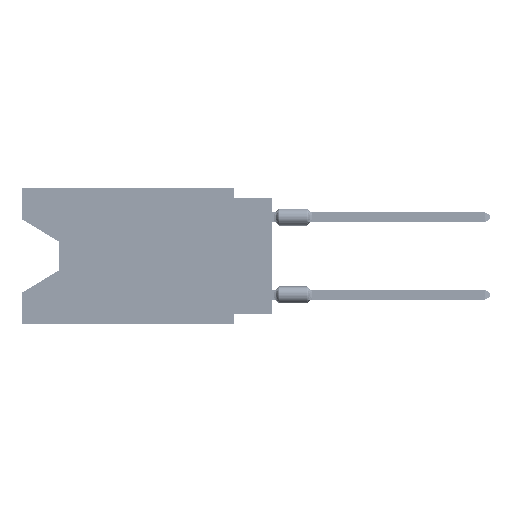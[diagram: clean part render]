
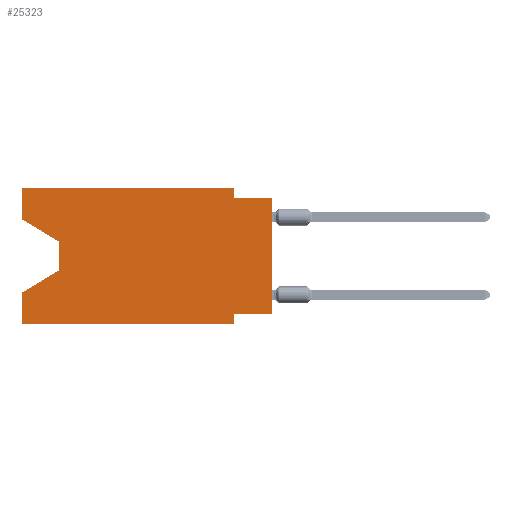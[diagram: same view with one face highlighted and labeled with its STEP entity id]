
A CAD part, left-side view. The second image highlights one B-rep face of the part: STEP entity #25323.
In plain terms, the highlighted planar face has unit normal (-1, 0, 0).
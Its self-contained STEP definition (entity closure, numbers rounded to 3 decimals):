
#1322 = DIRECTION ( 'NONE',  ( 0., -1., 0. ) ) ;
#2006 = CARTESIAN_POINT ( 'NONE',  ( 0., 2.54, -8.89 ) ) ;
#2215 = ORIENTED_EDGE ( 'NONE', *, *, #45818, .F. ) ;
#2625 = VECTOR ( 'NONE', #82214, 1000. ) ;
#3674 = CARTESIAN_POINT ( 'NONE',  ( 0., 16.383, -6.852 ) ) ;
#5440 = ORIENTED_EDGE ( 'NONE', *, *, #59265, .F. ) ;
#5467 = DIRECTION ( 'NONE',  ( 0., 0., -1. ) ) ;
#6270 = CARTESIAN_POINT ( 'NONE',  ( 0., 13.97, -3.505 ) ) ;
#6957 = VERTEX_POINT ( 'NONE', #6270 ) ;
#7101 = LINE ( 'NONE', #88736, #16648 ) ;
#7112 = LINE ( 'NONE', #82929, #27342 ) ;
#7454 = ORIENTED_EDGE ( 'NONE', *, *, #74596, .T. ) ;
#8491 = ORIENTED_EDGE ( 'NONE', *, *, #35704, .T. ) ;
#8925 = VERTEX_POINT ( 'NONE', #3674 ) ;
#10332 = CARTESIAN_POINT ( 'NONE',  ( 0., 16.383, -8.89 ) ) ;
#14227 = CARTESIAN_POINT ( 'NONE',  ( 0., 0., -8.255 ) ) ;
#15724 = VERTEX_POINT ( 'NONE', #23670 ) ;
#15824 = LINE ( 'NONE', #31757, #81781 ) ;
#16503 = LINE ( 'NONE', #47361, #63998 ) ;
#16648 = VECTOR ( 'NONE', #44758, 1000. ) ;
#17114 = ORIENTED_EDGE ( 'NONE', *, *, #38136, .F. ) ;
#20661 = ORIENTED_EDGE ( 'NONE', *, *, #65921, .T. ) ;
#21533 = EDGE_CURVE ( 'NONE', #89520, #93543, #53002, .T. ) ;
#22198 = ORIENTED_EDGE ( 'NONE', *, *, #42359, .F. ) ;
#23315 = EDGE_CURVE ( 'NONE', #33193, #8925, #7101, .T. ) ;
#23670 = CARTESIAN_POINT ( 'NONE',  ( 0., 16.383, 0. ) ) ;
#23879 = EDGE_LOOP ( 'NONE', ( #20661, #61763, #7454, #28850, #8491, #17114, #90145, #60807, #91221, #2215, #5440, #22198 ) ) ;
#24011 = DIRECTION ( 'NONE',  ( 0., 1., 0. ) ) ;
#24727 = VERTEX_POINT ( 'NONE', #70320 ) ;
#24990 = CARTESIAN_POINT ( 'NONE',  ( 0., 2.54, -8.255 ) ) ;
#25323 = ADVANCED_FACE ( 'NONE', ( #49422 ), #42177, .F. ) ;
#26216 = CARTESIAN_POINT ( 'NONE',  ( 0., 0., 0. ) ) ;
#27342 = VECTOR ( 'NONE', #24011, 1000. ) ;
#27748 = LINE ( 'NONE', #71210, #50982 ) ;
#28359 = VERTEX_POINT ( 'NONE', #14227 ) ;
#28481 = EDGE_CURVE ( 'NONE', #6957, #92949, #36915, .T. ) ;
#28850 = ORIENTED_EDGE ( 'NONE', *, *, #23315, .F. ) ;
#29168 = VECTOR ( 'NONE', #82790, 1000. ) ;
#29172 = AXIS2_PLACEMENT_3D ( 'NONE', #79857, #71643, #5467 ) ;
#31757 = CARTESIAN_POINT ( 'NONE',  ( 0., 16.383, 0. ) ) ;
#33193 = VERTEX_POINT ( 'NONE', #10332 ) ;
#35704 = EDGE_CURVE ( 'NONE', #33193, #24727, #16503, .T. ) ;
#36915 = LINE ( 'NONE', #51417, #29168 ) ;
#37193 = VECTOR ( 'NONE', #68085, 1000. ) ;
#38136 = EDGE_CURVE ( 'NONE', #65409, #24727, #59526, .T. ) ;
#38167 = LINE ( 'NONE', #45880, #37193 ) ;
#38247 = LINE ( 'NONE', #67692, #49862 ) ;
#38973 = CARTESIAN_POINT ( 'NONE',  ( 0., 0., -0.635 ) ) ;
#41274 = LINE ( 'NONE', #48996, #94945 ) ;
#42177 = PLANE ( 'NONE',  #29172 ) ;
#42359 = EDGE_CURVE ( 'NONE', #56810, #15724, #27748, .T. ) ;
#44758 = DIRECTION ( 'NONE',  ( 0., 0., 1. ) ) ;
#45664 = VECTOR ( 'NONE', #90646, 1000. ) ;
#45818 = EDGE_CURVE ( 'NONE', #68964, #89520, #38247, .T. ) ;
#45880 = CARTESIAN_POINT ( 'NONE',  ( 0., 13.97, -5.385 ) ) ;
#46516 = DIRECTION ( 'NONE',  ( 0., 0., 1. ) ) ;
#47361 = CARTESIAN_POINT ( 'NONE',  ( 0., 16.383, -8.89 ) ) ;
#47803 = CARTESIAN_POINT ( 'NONE',  ( 0., 16.383, -2.038 ) ) ;
#47938 = LINE ( 'NONE', #26216, #55516 ) ;
#48915 = CARTESIAN_POINT ( 'NONE',  ( 0., 13.97, -5.385 ) ) ;
#48996 = CARTESIAN_POINT ( 'NONE',  ( 0., 16.383, -2.038 ) ) ;
#49422 = FACE_OUTER_BOUND ( 'NONE', #23879, .T. ) ;
#49862 = VECTOR ( 'NONE', #56774, 1000. ) ;
#50982 = VECTOR ( 'NONE', #93420, 1000. ) ;
#51417 = CARTESIAN_POINT ( 'NONE',  ( 0., 13.97, -3.505 ) ) ;
#53002 = LINE ( 'NONE', #38973, #45664 ) ;
#55516 = VECTOR ( 'NONE', #46516, 1000. ) ;
#56774 = DIRECTION ( 'NONE',  ( 0., 0., -1. ) ) ;
#56810 = VERTEX_POINT ( 'NONE', #47803 ) ;
#57966 = EDGE_CURVE ( 'NONE', #28359, #93543, #47938, .T. ) ;
#59265 = EDGE_CURVE ( 'NONE', #15724, #68964, #15824, .T. ) ;
#59526 = LINE ( 'NONE', #2006, #2625 ) ;
#60807 = ORIENTED_EDGE ( 'NONE', *, *, #57966, .T. ) ;
#61763 = ORIENTED_EDGE ( 'NONE', *, *, #28481, .T. ) ;
#63998 = VECTOR ( 'NONE', #83140, 1000. ) ;
#65409 = VERTEX_POINT ( 'NONE', #24990 ) ;
#65921 = EDGE_CURVE ( 'NONE', #56810, #6957, #41274, .T. ) ;
#67692 = CARTESIAN_POINT ( 'NONE',  ( 0., 2.54, 0. ) ) ;
#68085 = DIRECTION ( 'NONE',  ( 0., 0.855, -0.519 ) ) ;
#68964 = VERTEX_POINT ( 'NONE', #72152 ) ;
#70320 = CARTESIAN_POINT ( 'NONE',  ( 0., 2.54, -8.89 ) ) ;
#71210 = CARTESIAN_POINT ( 'NONE',  ( 0., 16.383, 0. ) ) ;
#71643 = DIRECTION ( 'NONE',  ( 1., 0., 0. ) ) ;
#72152 = CARTESIAN_POINT ( 'NONE',  ( 0., 2.54, 0. ) ) ;
#74596 = EDGE_CURVE ( 'NONE', #92949, #8925, #38167, .T. ) ;
#79857 = CARTESIAN_POINT ( 'NONE',  ( 0., 16.383, 0. ) ) ;
#81178 = EDGE_CURVE ( 'NONE', #28359, #65409, #7112, .T. ) ;
#81781 = VECTOR ( 'NONE', #1322, 1000. ) ;
#82214 = DIRECTION ( 'NONE',  ( 0., 0., -1. ) ) ;
#82790 = DIRECTION ( 'NONE',  ( 0., 0., -1. ) ) ;
#82929 = CARTESIAN_POINT ( 'NONE',  ( 0., 0., -8.255 ) ) ;
#83140 = DIRECTION ( 'NONE',  ( 0., -1., 0. ) ) ;
#86182 = DIRECTION ( 'NONE',  ( 0., -0.855, -0.519 ) ) ;
#88736 = CARTESIAN_POINT ( 'NONE',  ( 0., 16.383, 0. ) ) ;
#89312 = CARTESIAN_POINT ( 'NONE',  ( 0., 0., -0.635 ) ) ;
#89520 = VERTEX_POINT ( 'NONE', #89639 ) ;
#89639 = CARTESIAN_POINT ( 'NONE',  ( 0., 2.54, -0.635 ) ) ;
#90145 = ORIENTED_EDGE ( 'NONE', *, *, #81178, .F. ) ;
#90646 = DIRECTION ( 'NONE',  ( 0., -1., 0. ) ) ;
#91221 = ORIENTED_EDGE ( 'NONE', *, *, #21533, .F. ) ;
#92949 = VERTEX_POINT ( 'NONE', #48915 ) ;
#93420 = DIRECTION ( 'NONE',  ( 0., 0., 1. ) ) ;
#93543 = VERTEX_POINT ( 'NONE', #89312 ) ;
#94945 = VECTOR ( 'NONE', #86182, 1000. ) ;
